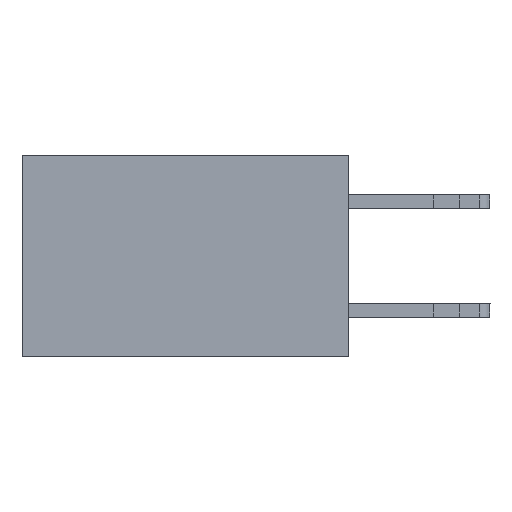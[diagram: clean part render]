
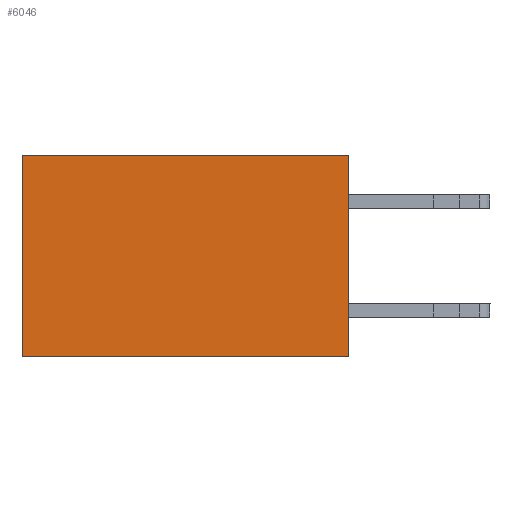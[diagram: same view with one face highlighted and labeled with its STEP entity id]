
A CAD part, left-side view. The second image highlights one B-rep face of the part: STEP entity #6046.
In plain terms, the highlighted planar face has unit normal (-1, 0, 0).
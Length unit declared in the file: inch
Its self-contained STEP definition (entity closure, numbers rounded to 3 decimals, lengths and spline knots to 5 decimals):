
#3 = VERTEX_POINT ( 'NONE', #18258 ) ;
#441 = CARTESIAN_POINT ( 'NONE',  ( 0.298, 0., -0.37 ) ) ;
#510 = CARTESIAN_POINT ( 'NONE',  ( 0.298, 0., 0. ) ) ;
#734 = VECTOR ( 'NONE', #12283, 39.37008 ) ;
#1277 = CARTESIAN_POINT ( 'NONE',  ( 0.298, 0.6, 0. ) ) ;
#1731 = VERTEX_POINT ( 'NONE', #13919 ) ;
#2530 = DIRECTION ( 'NONE',  ( 0., 0., -1. ) ) ;
#3918 = LINE ( 'NONE', #510, #7274 ) ;
#4082 = EDGE_CURVE ( 'NONE', #17176, #5610, #7742, .T. ) ;
#4826 = DIRECTION ( 'NONE',  ( 0., 0., -1. ) ) ;
#4960 = CARTESIAN_POINT ( 'NONE',  ( 0.298, 0., 0. ) ) ;
#5078 = VECTOR ( 'NONE', #15129, 39.37008 ) ;
#5610 = VERTEX_POINT ( 'NONE', #7683 ) ;
#6013 = FACE_OUTER_BOUND ( 'NONE', #17073, .T. ) ;
#6046 = ADVANCED_FACE ( 'NONE', ( #6013 ), #8037, .F. ) ;
#6160 = AXIS2_PLACEMENT_3D ( 'NONE', #4960, #7963, #4826 ) ;
#6544 = EDGE_CURVE ( 'NONE', #3, #1731, #10229, .T. ) ;
#7156 = VECTOR ( 'NONE', #2530, 39.37008 ) ;
#7274 = VECTOR ( 'NONE', #8031, 39.37008 ) ;
#7683 = CARTESIAN_POINT ( 'NONE',  ( 0.298, 0.6, -0.37 ) ) ;
#7742 = LINE ( 'NONE', #441, #734 ) ;
#7963 = DIRECTION ( 'NONE',  ( 1., 0., 0. ) ) ;
#8031 = DIRECTION ( 'NONE',  ( 0., 0., -1. ) ) ;
#8037 = PLANE ( 'NONE',  #6160 ) ;
#8162 = EDGE_CURVE ( 'NONE', #1731, #5610, #18337, .T. ) ;
#8259 = ORIENTED_EDGE ( 'NONE', *, *, #15180, .F. ) ;
#8951 = ORIENTED_EDGE ( 'NONE', *, *, #8162, .T. ) ;
#9787 = CARTESIAN_POINT ( 'NONE',  ( 0.298, 0., -0.37 ) ) ;
#10229 = LINE ( 'NONE', #10635, #5078 ) ;
#10635 = CARTESIAN_POINT ( 'NONE',  ( 0.298, 0., 0. ) ) ;
#12283 = DIRECTION ( 'NONE',  ( 0., 1., 0. ) ) ;
#13030 = ORIENTED_EDGE ( 'NONE', *, *, #4082, .F. ) ;
#13919 = CARTESIAN_POINT ( 'NONE',  ( 0.298, 0.6, 0. ) ) ;
#15129 = DIRECTION ( 'NONE',  ( 0., 1., 0. ) ) ;
#15180 = EDGE_CURVE ( 'NONE', #3, #17176, #3918, .T. ) ;
#17073 = EDGE_LOOP ( 'NONE', ( #8951, #13030, #8259, #17593 ) ) ;
#17176 = VERTEX_POINT ( 'NONE', #9787 ) ;
#17593 = ORIENTED_EDGE ( 'NONE', *, *, #6544, .T. ) ;
#18258 = CARTESIAN_POINT ( 'NONE',  ( 0.298, 0., 0. ) ) ;
#18337 = LINE ( 'NONE', #1277, #7156 ) ;
